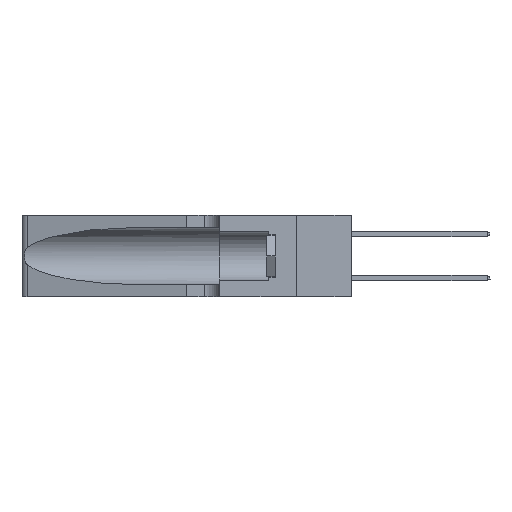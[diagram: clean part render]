
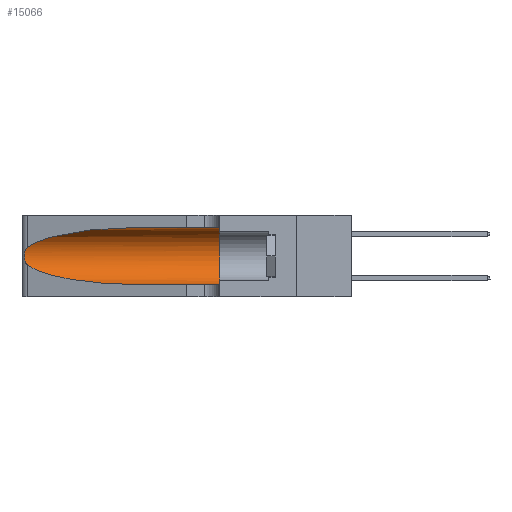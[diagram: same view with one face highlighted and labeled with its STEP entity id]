
A CAD part, left-side view. The second image highlights one B-rep face of the part: STEP entity #15066.
In plain terms, the highlighted cylindrical face has radius 3.308 mm (diameter 6.617 mm), a partial arc.
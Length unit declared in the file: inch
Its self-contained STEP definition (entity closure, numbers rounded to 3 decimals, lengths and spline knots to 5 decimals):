
#881 = DIRECTION ( 'NONE',  ( 0., 0., 1. ) ) ;
#1308 = CARTESIAN_POINT ( 'NONE',  ( 0.26075, 1.23896, 0.178 ) ) ;
#1370 = EDGE_CURVE ( 'NONE', #35200, #16274, #40714, .T. ) ;
#2334 = DIRECTION ( 'NONE',  ( 0., -1., 0. ) ) ;
#2676 = VERTEX_POINT ( 'NONE', #32329 ) ;
#3451 = VECTOR ( 'NONE', #2334, 39.37008 ) ;
#3702 = VERTEX_POINT ( 'NONE', #39361 ) ;
#4111 = CARTESIAN_POINT ( 'NONE',  ( 0.25639, 1.23184, 0.21858 ) ) ;
#5511 = LINE ( 'NONE', #40955, #3451 ) ;
#5677 = CARTESIAN_POINT ( 'NONE',  ( 0.2373, 1.15595, 0.28018 ) ) ;
#5770 = CYLINDRICAL_SURFACE ( 'NONE', #22330, 0.13025 ) ;
#7018 = ORIENTED_EDGE ( 'NONE', *, *, #23999, .F. ) ;
#7357 = CARTESIAN_POINT ( 'NONE',  ( 0.26017, 1.23833, 0.17102 ) ) ;
#7920 = CARTESIAN_POINT ( 'NONE',  ( 0.25856, 1.23593, 0.16098 ) ) ;
#9079 = CARTESIAN_POINT ( 'NONE',  ( 0.25487, 1.22718, 0.22369 ) ) ;
#10078 =( BOUNDED_CURVE ( )  B_SPLINE_CURVE ( 3, ( #15609, #37980, #5677, #9079 ),
 .UNSPECIFIED., .F., .F. ) 
 B_SPLINE_CURVE_WITH_KNOTS ( ( 4, 4 ),
 ( 1.5708, 2.84003 ),
 .UNSPECIFIED. ) 
 CURVE ( )  GEOMETRIC_REPRESENTATION_ITEM ( )  RATIONAL_B_SPLINE_CURVE ( ( 1., 0.87, 0.87, 1. ) ) 
 REPRESENTATION_ITEM ( '' )  );
#10896 = CARTESIAN_POINT ( 'NONE',  ( 0.25555, 1.22994, 0.2215 ) ) ;
#12588 = CARTESIAN_POINT ( 'NONE',  ( 0.18966, 0.96281, 0.05475 ) ) ;
#12723 = CARTESIAN_POINT ( 'NONE',  ( 0.25487, 1.22718, 0.14631 ) ) ;
#12956 = CIRCLE ( 'NONE', #18506, 0.13025 ) ;
#13732 = CARTESIAN_POINT ( 'NONE',  ( 0.25787, 1.23484, 0.2124 ) ) ;
#14404 = FACE_OUTER_BOUND ( 'NONE', #29314, .T. ) ;
#14667 = DIRECTION ( 'NONE',  ( 0., -1., 0. ) ) ;
#15066 = ADVANCED_FACE ( 'NONE', ( #14404 ), #5770, .F. ) ;
#15082 =( BOUNDED_CURVE ( )  B_SPLINE_CURVE ( 3, ( #12723, #16280, #12588, #38651 ),
 .UNSPECIFIED., .F., .T. ) 
 B_SPLINE_CURVE_WITH_KNOTS ( ( 4, 4 ),
 ( 3.44316, 4.71239 ),
 .UNSPECIFIED. ) 
 CURVE ( )  GEOMETRIC_REPRESENTATION_ITEM ( )  RATIONAL_B_SPLINE_CURVE ( ( 1., 0.87, 0.87, 1. ) ) 
 REPRESENTATION_ITEM ( '' )  );
#15609 = CARTESIAN_POINT ( 'NONE',  ( 0.1305, 0.72297, 0.31525 ) ) ;
#15972 = ORIENTED_EDGE ( 'NONE', *, *, #38636, .T. ) ;
#16274 = VERTEX_POINT ( 'NONE', #20269 ) ;
#16280 = CARTESIAN_POINT ( 'NONE',  ( 0.2373, 1.15595, 0.08982 ) ) ;
#16971 = CARTESIAN_POINT ( 'NONE',  ( 0.25555, 1.22993, 0.14849 ) ) ;
#17350 = CARTESIAN_POINT ( 'NONE',  ( 0.1305, 1.61858, 0.31525 ) ) ;
#17421 = CARTESIAN_POINT ( 'NONE',  ( 0.25639, 1.23186, 0.15144 ) ) ;
#17609 = VECTOR ( 'NONE', #14667, 39.37008 ) ;
#18506 = AXIS2_PLACEMENT_3D ( 'NONE', #35504, #26565, #881 ) ;
#20269 = CARTESIAN_POINT ( 'NONE',  ( 0.1305, 0.35, 0.31525 ) ) ;
#20380 = CARTESIAN_POINT ( 'NONE',  ( 0.26075, 1.23896, 0.19203 ) ) ;
#21003 = EDGE_CURVE ( 'NONE', #2676, #3702, #38807, .T. ) ;
#22197 = VERTEX_POINT ( 'NONE', #38347 ) ;
#22330 = AXIS2_PLACEMENT_3D ( 'NONE', #37125, #24218, #27001 ) ;
#23635 = CARTESIAN_POINT ( 'NONE',  ( 0.25789, 1.23486, 0.15765 ) ) ;
#23999 = EDGE_CURVE ( 'NONE', #16274, #34948, #12956, .T. ) ;
#24218 = DIRECTION ( 'NONE',  ( 0., -1., 0. ) ) ;
#26565 = DIRECTION ( 'NONE',  ( 0., 1., 0. ) ) ;
#27001 = DIRECTION ( 'NONE',  ( 0., 0., -1. ) ) ;
#27406 = CARTESIAN_POINT ( 'NONE',  ( 0.1305, 0.72297, 0.31525 ) ) ;
#29272 = EDGE_CURVE ( 'NONE', #22197, #34948, #5511, .T. ) ;
#29314 = EDGE_LOOP ( 'NONE', ( #34967, #30053, #15972, #37193, #7018, #37488 ) ) ;
#29812 = CARTESIAN_POINT ( 'NONE',  ( 0.1305, 0.35, 0.05475 ) ) ;
#29966 = CARTESIAN_POINT ( 'NONE',  ( 0.25487, 1.22718, 0.14631 ) ) ;
#30053 = ORIENTED_EDGE ( 'NONE', *, *, #21003, .T. ) ;
#32329 = CARTESIAN_POINT ( 'NONE',  ( 0.25487, 1.22718, 0.22369 ) ) ;
#34787 = EDGE_CURVE ( 'NONE', #35200, #2676, #10078, .T. ) ;
#34948 = VERTEX_POINT ( 'NONE', #29812 ) ;
#34967 = ORIENTED_EDGE ( 'NONE', *, *, #34787, .T. ) ;
#35200 = VERTEX_POINT ( 'NONE', #27406 ) ;
#35504 = CARTESIAN_POINT ( 'NONE',  ( 0.1305, 0.35, 0.185 ) ) ;
#36300 = CARTESIAN_POINT ( 'NONE',  ( 0.26018, 1.23835, 0.19895 ) ) ;
#37125 = CARTESIAN_POINT ( 'NONE',  ( 0.1305, 1.61858, 0.185 ) ) ;
#37193 = ORIENTED_EDGE ( 'NONE', *, *, #29272, .T. ) ;
#37488 = ORIENTED_EDGE ( 'NONE', *, *, #1370, .F. ) ;
#37980 = CARTESIAN_POINT ( 'NONE',  ( 0.18966, 0.96281, 0.31525 ) ) ;
#38347 = CARTESIAN_POINT ( 'NONE',  ( 0.1305, 0.72297, 0.05475 ) ) ;
#38636 = EDGE_CURVE ( 'NONE', #3702, #22197, #15082, .T. ) ;
#38651 = CARTESIAN_POINT ( 'NONE',  ( 0.1305, 0.72297, 0.05475 ) ) ;
#38807 = B_SPLINE_CURVE_WITH_KNOTS ( 'NONE', 3,
 ( #40087, #10896, #4111, #13732, #39642, #36300, #20380, #1308, #7357, #7920, #23635, #17421, #16971, #29966 ),
 .UNSPECIFIED., .F., .F.,
 ( 4, 2, 2, 2, 2, 2, 4 ),
 ( 0., 0.00027, 0.00053, 0.00107, 0.0016, 0.00187, 0.00214 ),
 .UNSPECIFIED. ) ;
#39361 = CARTESIAN_POINT ( 'NONE',  ( 0.25487, 1.22718, 0.14631 ) ) ;
#39642 = CARTESIAN_POINT ( 'NONE',  ( 0.25854, 1.2359, 0.20912 ) ) ;
#40087 = CARTESIAN_POINT ( 'NONE',  ( 0.25487, 1.22718, 0.22369 ) ) ;
#40714 = LINE ( 'NONE', #17350, #17609 ) ;
#40955 = CARTESIAN_POINT ( 'NONE',  ( 0.1305, 1.61858, 0.05475 ) ) ;
